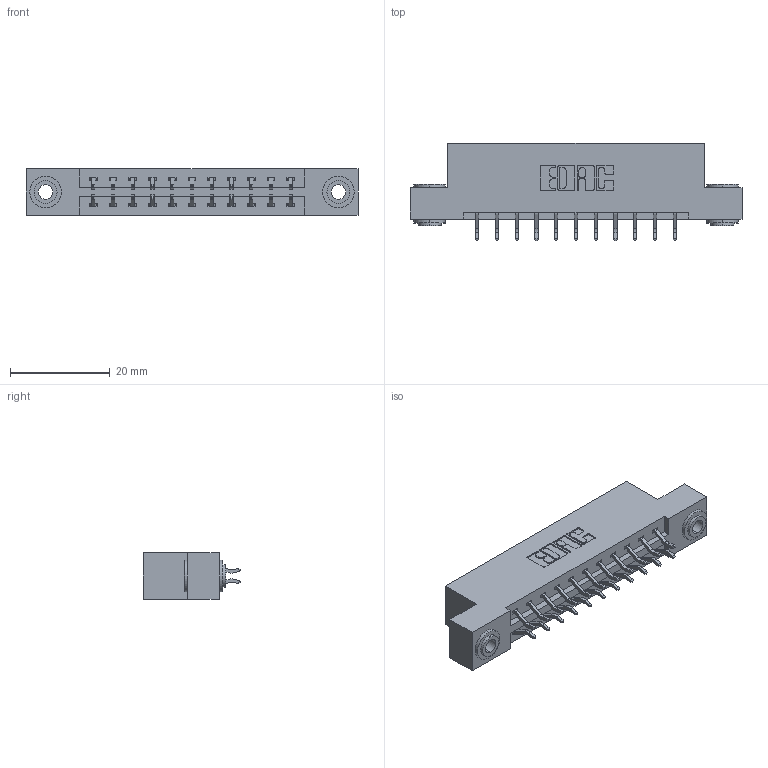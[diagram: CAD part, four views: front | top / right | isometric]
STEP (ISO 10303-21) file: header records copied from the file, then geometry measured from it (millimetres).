
FILE_DESCRIPTION (( 'STEP AP203' ), '1' );
FILE_NAME ('387-022-556-203.STEP', '2018-09-14T06:00:40', ( '' ), ( '' ), 'SwSTEP 2.0', 'SolidWorks 2016', '' );
FILE_SCHEMA (( 'CONFIG_CONTROL_DESIGN' ));
Length unit declared in the file: inch
Products named in the file (4): 337 Part_Flush Mounting Lugs - 0.156 Dia-TH; 345-292-001_556 Tail; 345-250-002_345-250-002-102; 387-022-556-203
Assembly tree (25 placements, depth 2):
  387-022-556-203
    337 Part_Flush Mounting Lugs - 0.156 Dia-TH
    345-292-001_556 Tail  x22
    345-250-002_345-250-002-102  x2
Bounding box: 66.6 x 19.57 x 9.4 mm (x, y, z)
Volume: 6624.6 mm3; surface area: 7389.2 mm2
Topology: 25 solids, 25 shells, 1472 faces, 4325 edges, 2850 vertices
Faces by surface type: plane 1004, cylinder 460, cone 8
Entity records: 13408 total; most frequent: CARTESIAN_POINT 2273, ORIENTED_EDGE 2190, DIRECTION 2013, EDGE_CURVE 1095, LINE 935, VECTOR 935, VERTEX_POINT 726, AXIS2_PLACEMENT_3D 539
